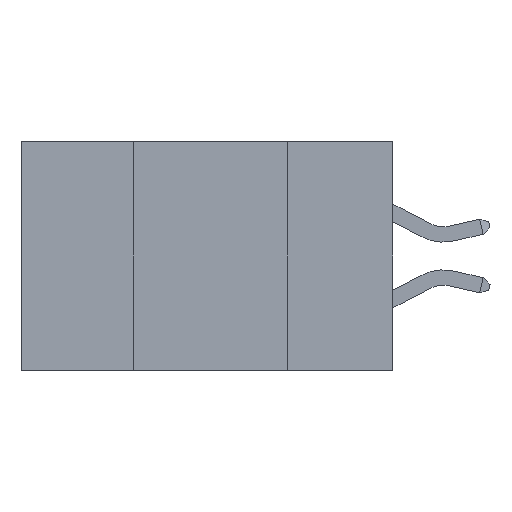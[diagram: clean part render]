
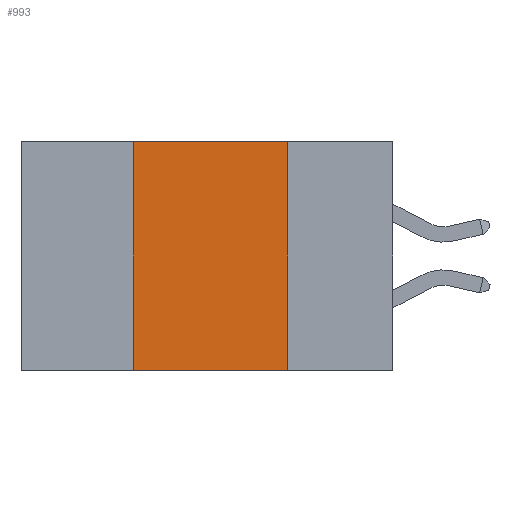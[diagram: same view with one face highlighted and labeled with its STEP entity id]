
A CAD part, left-side view. The second image highlights one B-rep face of the part: STEP entity #993.
In plain terms, the highlighted planar face has unit normal (-1, 0, 0).
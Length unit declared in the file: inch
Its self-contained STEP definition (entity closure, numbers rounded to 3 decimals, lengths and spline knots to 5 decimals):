
#228 = FACE_OUTER_BOUND ( 'NONE', #14969, .T. ) ;
#993 = ADVANCED_FACE ( 'NONE', ( #228 ), #16916, .F. ) ;
#1487 = VERTEX_POINT ( 'NONE', #18211 ) ;
#1577 = CARTESIAN_POINT ( 'NONE',  ( 0., 0.6, 0. ) ) ;
#1717 = CARTESIAN_POINT ( 'NONE',  ( 0., 0.6, -0.37 ) ) ;
#1818 = ORIENTED_EDGE ( 'NONE', *, *, #19645, .F. ) ;
#2521 = DIRECTION ( 'NONE',  ( 0., 0., -1. ) ) ;
#3679 = DIRECTION ( 'NONE',  ( 0., -1., 0. ) ) ;
#4712 = AXIS2_PLACEMENT_3D ( 'NONE', #23086, #8158, #2521 ) ;
#5813 = LINE ( 'NONE', #1577, #15117 ) ;
#8158 = DIRECTION ( 'NONE',  ( 1., 0., 0. ) ) ;
#8691 = VERTEX_POINT ( 'NONE', #13411 ) ;
#9734 = DIRECTION ( 'NONE',  ( 0., 0., -1. ) ) ;
#10226 = EDGE_CURVE ( 'NONE', #12386, #13982, #24611, .T. ) ;
#11821 = CARTESIAN_POINT ( 'NONE',  ( 0., 0.17, 0. ) ) ;
#12386 = VERTEX_POINT ( 'NONE', #22297 ) ;
#12733 = ORIENTED_EDGE ( 'NONE', *, *, #23823, .F. ) ;
#13411 = CARTESIAN_POINT ( 'NONE',  ( 0., 0.17, 0. ) ) ;
#13982 = VERTEX_POINT ( 'NONE', #18918 ) ;
#13989 = DIRECTION ( 'NONE',  ( 0., 0., 1. ) ) ;
#14969 = EDGE_LOOP ( 'NONE', ( #20234, #1818, #12733, #16609 ) ) ;
#15117 = VECTOR ( 'NONE', #3679, 39.37008 ) ;
#15896 = CARTESIAN_POINT ( 'NONE',  ( 0., 0.42, 0. ) ) ;
#16609 = ORIENTED_EDGE ( 'NONE', *, *, #10226, .T. ) ;
#16632 = VECTOR ( 'NONE', #22106, 39.37008 ) ;
#16916 = PLANE ( 'NONE',  #4712 ) ;
#17801 = EDGE_CURVE ( 'NONE', #8691, #13982, #21961, .T. ) ;
#18211 = CARTESIAN_POINT ( 'NONE',  ( 0., 0.42, 0. ) ) ;
#18918 = CARTESIAN_POINT ( 'NONE',  ( 0., 0.17, -0.37 ) ) ;
#19184 = VECTOR ( 'NONE', #9734, 39.37008 ) ;
#19645 = EDGE_CURVE ( 'NONE', #1487, #8691, #5813, .T. ) ;
#20234 = ORIENTED_EDGE ( 'NONE', *, *, #17801, .F. ) ;
#20852 = LINE ( 'NONE', #15896, #23616 ) ;
#21961 = LINE ( 'NONE', #11821, #19184 ) ;
#22106 = DIRECTION ( 'NONE',  ( 0., -1., 0. ) ) ;
#22297 = CARTESIAN_POINT ( 'NONE',  ( 0., 0.42, -0.37 ) ) ;
#23086 = CARTESIAN_POINT ( 'NONE',  ( 0., 0.6, 0. ) ) ;
#23616 = VECTOR ( 'NONE', #13989, 39.37008 ) ;
#23823 = EDGE_CURVE ( 'NONE', #12386, #1487, #20852, .T. ) ;
#24611 = LINE ( 'NONE', #1717, #16632 ) ;
